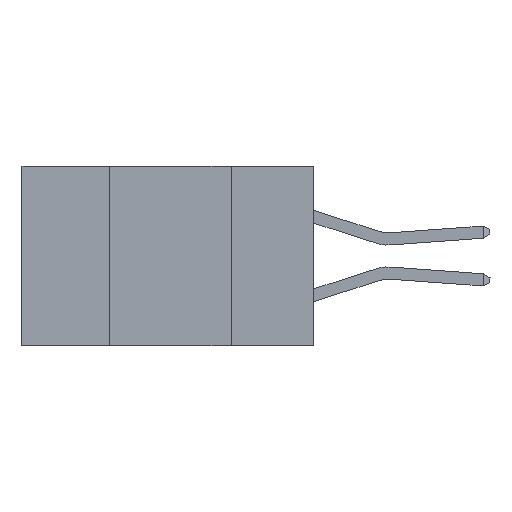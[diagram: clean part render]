
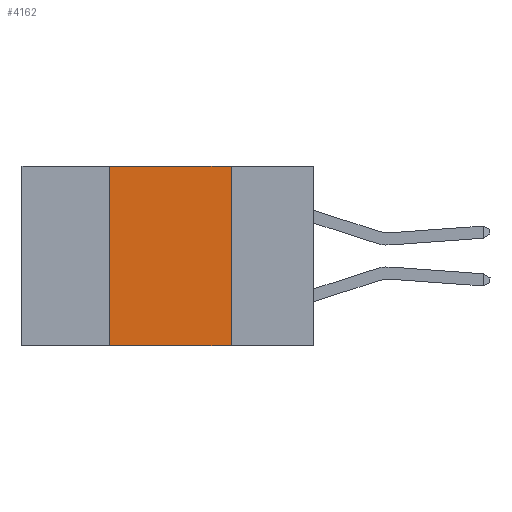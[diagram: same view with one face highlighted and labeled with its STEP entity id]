
A CAD part, left-side view. The second image highlights one B-rep face of the part: STEP entity #4162.
In plain terms, the highlighted planar face has unit normal (-1, 0, 0).
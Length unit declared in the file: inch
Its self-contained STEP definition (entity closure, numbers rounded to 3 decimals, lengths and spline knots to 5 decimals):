
#541 = ORIENTED_EDGE ( 'NONE', *, *, #29940, .F. ) ;
#1281 = LINE ( 'NONE', #18539, #27360 ) ;
#1678 = CARTESIAN_POINT ( 'NONE',  ( 0., 0.42, 0. ) ) ;
#2154 = CARTESIAN_POINT ( 'NONE',  ( 0., 0.17, 0. ) ) ;
#2374 = AXIS2_PLACEMENT_3D ( 'NONE', #22265, #5151, #24335 ) ;
#3095 = VERTEX_POINT ( 'NONE', #4014 ) ;
#3156 = CARTESIAN_POINT ( 'NONE',  ( 0., 0.17, 0. ) ) ;
#4014 = CARTESIAN_POINT ( 'NONE',  ( 0., 0.42, 0. ) ) ;
#4033 = LINE ( 'NONE', #1678, #18202 ) ;
#4162 = ADVANCED_FACE ( 'NONE', ( #7338 ), #21639, .F. ) ;
#4306 = CARTESIAN_POINT ( 'NONE',  ( 0., 0.17, -0.37 ) ) ;
#4869 = VECTOR ( 'NONE', #28201, 39.37008 ) ;
#5151 = DIRECTION ( 'NONE',  ( 1., 0., 0. ) ) ;
#5392 = EDGE_CURVE ( 'NONE', #17002, #18487, #19309, .T. ) ;
#6541 = VERTEX_POINT ( 'NONE', #18404 ) ;
#7338 = FACE_OUTER_BOUND ( 'NONE', #17785, .T. ) ;
#9360 = LINE ( 'NONE', #18973, #4869 ) ;
#16318 = ORIENTED_EDGE ( 'NONE', *, *, #26577, .F. ) ;
#16937 = DIRECTION ( 'NONE',  ( 0., 0., -1. ) ) ;
#17002 = VERTEX_POINT ( 'NONE', #3156 ) ;
#17482 = ORIENTED_EDGE ( 'NONE', *, *, #24024, .T. ) ;
#17785 = EDGE_LOOP ( 'NONE', ( #19762, #541, #16318, #17482 ) ) ;
#18202 = VECTOR ( 'NONE', #28056, 39.37008 ) ;
#18404 = CARTESIAN_POINT ( 'NONE',  ( 0., 0.42, -0.37 ) ) ;
#18487 = VERTEX_POINT ( 'NONE', #4306 ) ;
#18539 = CARTESIAN_POINT ( 'NONE',  ( 0., 0.6, 0. ) ) ;
#18973 = CARTESIAN_POINT ( 'NONE',  ( 0., 0.6, -0.37 ) ) ;
#19309 = LINE ( 'NONE', #2154, #21702 ) ;
#19762 = ORIENTED_EDGE ( 'NONE', *, *, #5392, .F. ) ;
#21639 = PLANE ( 'NONE',  #2374 ) ;
#21702 = VECTOR ( 'NONE', #16937, 39.37008 ) ;
#22265 = CARTESIAN_POINT ( 'NONE',  ( 0., 0.6, 0. ) ) ;
#24024 = EDGE_CURVE ( 'NONE', #6541, #18487, #9360, .T. ) ;
#24335 = DIRECTION ( 'NONE',  ( 0., 0., -1. ) ) ;
#26577 = EDGE_CURVE ( 'NONE', #6541, #3095, #4033, .T. ) ;
#27360 = VECTOR ( 'NONE', #29546, 39.37008 ) ;
#28056 = DIRECTION ( 'NONE',  ( 0., 0., 1. ) ) ;
#28201 = DIRECTION ( 'NONE',  ( 0., -1., 0. ) ) ;
#29546 = DIRECTION ( 'NONE',  ( 0., -1., 0. ) ) ;
#29940 = EDGE_CURVE ( 'NONE', #3095, #17002, #1281, .T. ) ;
